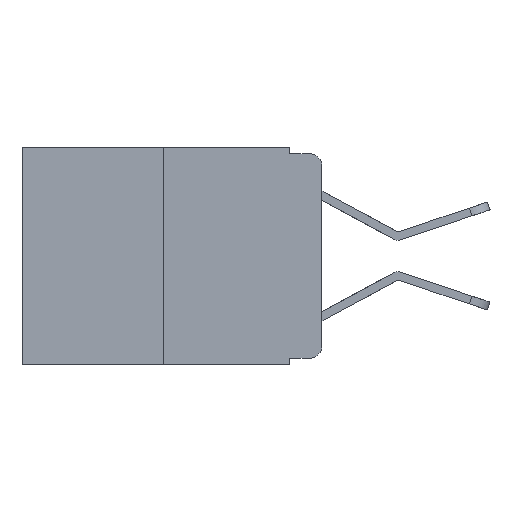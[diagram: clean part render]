
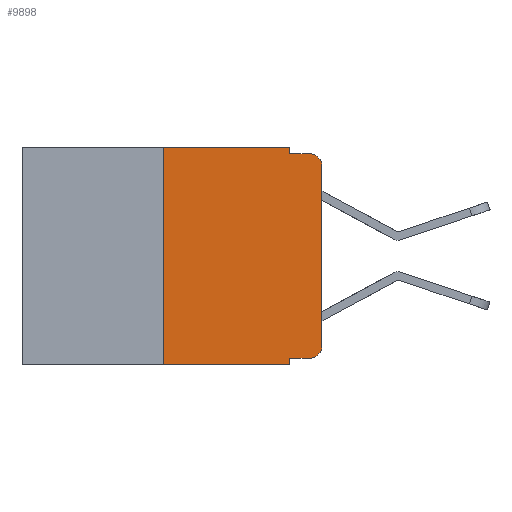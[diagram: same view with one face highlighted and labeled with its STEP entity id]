
A CAD part, left-side view. The second image highlights one B-rep face of the part: STEP entity #9898.
In plain terms, the highlighted planar face has unit normal (-1, 0, 0).
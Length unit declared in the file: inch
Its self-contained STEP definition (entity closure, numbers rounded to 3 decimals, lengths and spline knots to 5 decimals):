
#82 = CARTESIAN_POINT ( 'NONE',  ( 0., 0.051, 0. ) ) ;
#129 = CARTESIAN_POINT ( 'NONE',  ( 0., 0.051, -0.01 ) ) ;
#152 = VECTOR ( 'NONE', #2446, 39.37008 ) ;
#193 = CARTESIAN_POINT ( 'NONE',  ( 0., 0.473, -0.343 ) ) ;
#271 = AXIS2_PLACEMENT_3D ( 'NONE', #11330, #11258, #11253 ) ;
#404 = CARTESIAN_POINT ( 'NONE',  ( 0., 0.051, -0.333 ) ) ;
#431 = CARTESIAN_POINT ( 'NONE',  ( 0., 0.051, 0. ) ) ;
#445 = ORIENTED_EDGE ( 'NONE', *, *, #9024, .F. ) ;
#812 = VECTOR ( 'NONE', #2411, 39.37008 ) ;
#1023 = CARTESIAN_POINT ( 'NONE',  ( 0., 0.25, 0. ) ) ;
#1127 = LINE ( 'NONE', #431, #812 ) ;
#1175 = DIRECTION ( 'NONE',  ( 0., 0., 1. ) ) ;
#1439 = ORIENTED_EDGE ( 'NONE', *, *, #10359, .F. ) ;
#1575 = EDGE_CURVE ( 'NONE', #4896, #1984, #9086, .T. ) ;
#1619 = EDGE_LOOP ( 'NONE', ( #9173, #3023, #445, #6154, #1943, #9426, #5337, #1439, #6356, #2566 ) ) ;
#1701 = AXIS2_PLACEMENT_3D ( 'NONE', #5255, #11457, #6163 ) ;
#1853 = DIRECTION ( 'NONE',  ( 1., 0., 0. ) ) ;
#1867 = DIRECTION ( 'NONE',  ( 0., -1., 0. ) ) ;
#1943 = ORIENTED_EDGE ( 'NONE', *, *, #9428, .F. ) ;
#1984 = VERTEX_POINT ( 'NONE', #8730 ) ;
#2051 = LINE ( 'NONE', #129, #9165 ) ;
#2201 = LINE ( 'NONE', #193, #9289 ) ;
#2274 = VERTEX_POINT ( 'NONE', #4433 ) ;
#2411 = DIRECTION ( 'NONE',  ( 0., 0., -1. ) ) ;
#2446 = DIRECTION ( 'NONE',  ( 0., 0., 1. ) ) ;
#2449 = AXIS2_PLACEMENT_3D ( 'NONE', #11837, #1853, #8398 ) ;
#2556 = VERTEX_POINT ( 'NONE', #6078 ) ;
#2566 = ORIENTED_EDGE ( 'NONE', *, *, #7800, .T. ) ;
#2801 = LINE ( 'NONE', #5280, #152 ) ;
#2817 = EDGE_CURVE ( 'NONE', #6727, #8221, #5365, .T. ) ;
#2953 = CARTESIAN_POINT ( 'NONE',  ( 0., 0.25, -0.343 ) ) ;
#3023 = ORIENTED_EDGE ( 'NONE', *, *, #1575, .T. ) ;
#3147 = VERTEX_POINT ( 'NONE', #2953 ) ;
#3574 = VERTEX_POINT ( 'NONE', #11815 ) ;
#3961 = LINE ( 'NONE', #6858, #6142 ) ;
#4314 = CARTESIAN_POINT ( 'NONE',  ( 0., 0.051, 0. ) ) ;
#4433 = CARTESIAN_POINT ( 'NONE',  ( 0., 0.051, -0.01 ) ) ;
#4495 = CARTESIAN_POINT ( 'NONE',  ( 0., 0.051, -0.333 ) ) ;
#4631 = DIRECTION ( 'NONE',  ( 0., -1., 0. ) ) ;
#4762 = CIRCLE ( 'NONE', #1701, 0.02 ) ;
#4896 = VERTEX_POINT ( 'NONE', #9828 ) ;
#5017 = DIRECTION ( 'NONE',  ( 0., -1., 0. ) ) ;
#5032 = DIRECTION ( 'NONE',  ( 0., -1., 0. ) ) ;
#5069 = VECTOR ( 'NONE', #1867, 39.37008 ) ;
#5255 = CARTESIAN_POINT ( 'NONE',  ( 0., 0.02, -0.313 ) ) ;
#5274 = DIRECTION ( 'NONE',  ( 0., 0., -1. ) ) ;
#5280 = CARTESIAN_POINT ( 'NONE',  ( 0., 0.25, 0. ) ) ;
#5337 = ORIENTED_EDGE ( 'NONE', *, *, #8270, .T. ) ;
#5365 = LINE ( 'NONE', #404, #5069 ) ;
#5436 = EDGE_CURVE ( 'NONE', #3147, #7174, #2801, .T. ) ;
#6030 = FACE_OUTER_BOUND ( 'NONE', #1619, .T. ) ;
#6078 = CARTESIAN_POINT ( 'NONE',  ( 0., 0., -0.313 ) ) ;
#6142 = VECTOR ( 'NONE', #1175, 39.37008 ) ;
#6154 = ORIENTED_EDGE ( 'NONE', *, *, #9585, .F. ) ;
#6163 = DIRECTION ( 'NONE',  ( 0., 0., -1. ) ) ;
#6356 = ORIENTED_EDGE ( 'NONE', *, *, #2817, .T. ) ;
#6727 = VERTEX_POINT ( 'NONE', #4495 ) ;
#6858 = CARTESIAN_POINT ( 'NONE',  ( 0., 0., 0. ) ) ;
#6892 = LINE ( 'NONE', #4314, #8728 ) ;
#7174 = VERTEX_POINT ( 'NONE', #1023 ) ;
#7381 = CARTESIAN_POINT ( 'NONE',  ( 0., 0.473, 0. ) ) ;
#7719 = CARTESIAN_POINT ( 'NONE',  ( 0., 0.02, -0.333 ) ) ;
#7800 = EDGE_CURVE ( 'NONE', #8221, #2556, #4762, .T. ) ;
#8221 = VERTEX_POINT ( 'NONE', #7719 ) ;
#8270 = EDGE_CURVE ( 'NONE', #3147, #3574, #2201, .T. ) ;
#8398 = DIRECTION ( 'NONE',  ( 0., 0., -1. ) ) ;
#8728 = VECTOR ( 'NONE', #5274, 39.37008 ) ;
#8730 = CARTESIAN_POINT ( 'NONE',  ( 0., 0.02, -0.01 ) ) ;
#9024 = EDGE_CURVE ( 'NONE', #2274, #1984, #2051, .T. ) ;
#9086 = CIRCLE ( 'NONE', #271, 0.02 ) ;
#9165 = VECTOR ( 'NONE', #5017, 39.37008 ) ;
#9173 = ORIENTED_EDGE ( 'NONE', *, *, #11656, .T. ) ;
#9289 = VECTOR ( 'NONE', #5032, 39.37008 ) ;
#9426 = ORIENTED_EDGE ( 'NONE', *, *, #5436, .F. ) ;
#9428 = EDGE_CURVE ( 'NONE', #7174, #10912, #9956, .T. ) ;
#9585 = EDGE_CURVE ( 'NONE', #10912, #2274, #1127, .T. ) ;
#9828 = CARTESIAN_POINT ( 'NONE',  ( 0., 0., -0.03 ) ) ;
#9898 = ADVANCED_FACE ( 'NONE', ( #6030 ), #10094, .F. ) ;
#9956 = LINE ( 'NONE', #7381, #10496 ) ;
#10094 = PLANE ( 'NONE',  #2449 ) ;
#10359 = EDGE_CURVE ( 'NONE', #6727, #3574, #6892, .T. ) ;
#10496 = VECTOR ( 'NONE', #4631, 39.37008 ) ;
#10912 = VERTEX_POINT ( 'NONE', #82 ) ;
#11253 = DIRECTION ( 'NONE',  ( 0., 0., -1. ) ) ;
#11258 = DIRECTION ( 'NONE',  ( -1., 0., 0. ) ) ;
#11330 = CARTESIAN_POINT ( 'NONE',  ( 0., 0.02, -0.03 ) ) ;
#11457 = DIRECTION ( 'NONE',  ( -1., 0., 0. ) ) ;
#11656 = EDGE_CURVE ( 'NONE', #2556, #4896, #3961, .T. ) ;
#11815 = CARTESIAN_POINT ( 'NONE',  ( 0., 0.051, -0.343 ) ) ;
#11837 = CARTESIAN_POINT ( 'NONE',  ( 0., 0.473, 0. ) ) ;
